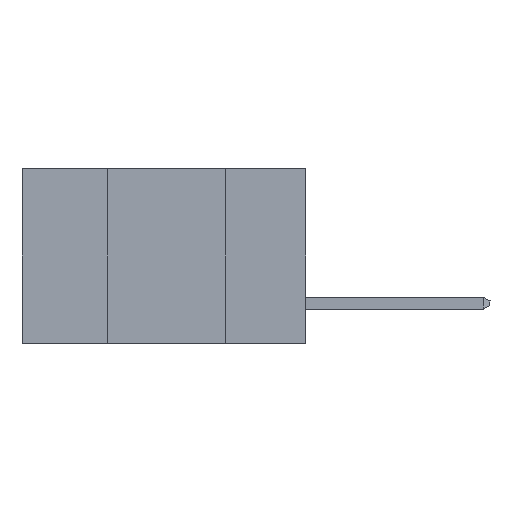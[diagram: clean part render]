
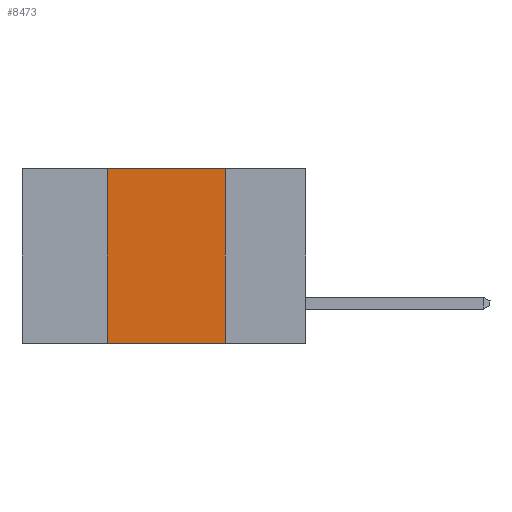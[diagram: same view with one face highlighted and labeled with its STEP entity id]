
A CAD part, left-side view. The second image highlights one B-rep face of the part: STEP entity #8473.
In plain terms, the highlighted planar face has unit normal (-1, 0, 0).
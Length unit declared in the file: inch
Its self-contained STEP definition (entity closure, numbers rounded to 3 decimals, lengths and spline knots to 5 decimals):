
#187 = CARTESIAN_POINT ( 'NONE',  ( 0., 0.6, -0.37 ) ) ;
#443 = DIRECTION ( 'NONE',  ( 1., 0., 0. ) ) ;
#593 = CARTESIAN_POINT ( 'NONE',  ( 0., 0.42, 0. ) ) ;
#1266 = DIRECTION ( 'NONE',  ( 0., 0., -1. ) ) ;
#4427 = ORIENTED_EDGE ( 'NONE', *, *, #7459, .F. ) ;
#4487 = VERTEX_POINT ( 'NONE', #4599 ) ;
#4599 = CARTESIAN_POINT ( 'NONE',  ( 0., 0.42, -0.37 ) ) ;
#4730 = VERTEX_POINT ( 'NONE', #4933 ) ;
#4838 = DIRECTION ( 'NONE',  ( 0., 0., 1. ) ) ;
#4933 = CARTESIAN_POINT ( 'NONE',  ( 0., 0.17, -0.37 ) ) ;
#4942 = ORIENTED_EDGE ( 'NONE', *, *, #14168, .F. ) ;
#4955 = LINE ( 'NONE', #593, #17452 ) ;
#6297 = VECTOR ( 'NONE', #11266, 39.37008 ) ;
#6928 = FACE_OUTER_BOUND ( 'NONE', #7159, .T. ) ;
#7159 = EDGE_LOOP ( 'NONE', ( #4942, #14814, #4427, #17120 ) ) ;
#7428 = DIRECTION ( 'NONE',  ( 0., 0., -1. ) ) ;
#7459 = EDGE_CURVE ( 'NONE', #4487, #10623, #4955, .T. ) ;
#8473 = ADVANCED_FACE ( 'NONE', ( #6928 ), #11521, .F. ) ;
#10623 = VERTEX_POINT ( 'NONE', #15572 ) ;
#10651 = DIRECTION ( 'NONE',  ( 0., -1., 0. ) ) ;
#11023 = LINE ( 'NONE', #12219, #14434 ) ;
#11266 = DIRECTION ( 'NONE',  ( 0., -1., 0. ) ) ;
#11521 = PLANE ( 'NONE',  #16994 ) ;
#12219 = CARTESIAN_POINT ( 'NONE',  ( 0., 0.17, 0. ) ) ;
#12775 = CARTESIAN_POINT ( 'NONE',  ( 0., 0.6, 0. ) ) ;
#13540 = EDGE_CURVE ( 'NONE', #4487, #4730, #14894, .T. ) ;
#13629 = CARTESIAN_POINT ( 'NONE',  ( 0., 0.17, 0. ) ) ;
#14168 = EDGE_CURVE ( 'NONE', #14519, #4730, #11023, .T. ) ;
#14434 = VECTOR ( 'NONE', #1266, 39.37008 ) ;
#14519 = VERTEX_POINT ( 'NONE', #13629 ) ;
#14814 = ORIENTED_EDGE ( 'NONE', *, *, #17573, .F. ) ;
#14894 = LINE ( 'NONE', #187, #6297 ) ;
#15572 = CARTESIAN_POINT ( 'NONE',  ( 0., 0.42, 0. ) ) ;
#16235 = CARTESIAN_POINT ( 'NONE',  ( 0., 0.6, 0. ) ) ;
#16641 = VECTOR ( 'NONE', #10651, 39.37008 ) ;
#16841 = LINE ( 'NONE', #16235, #16641 ) ;
#16994 = AXIS2_PLACEMENT_3D ( 'NONE', #12775, #443, #7428 ) ;
#17120 = ORIENTED_EDGE ( 'NONE', *, *, #13540, .T. ) ;
#17452 = VECTOR ( 'NONE', #4838, 39.37008 ) ;
#17573 = EDGE_CURVE ( 'NONE', #10623, #14519, #16841, .T. ) ;
